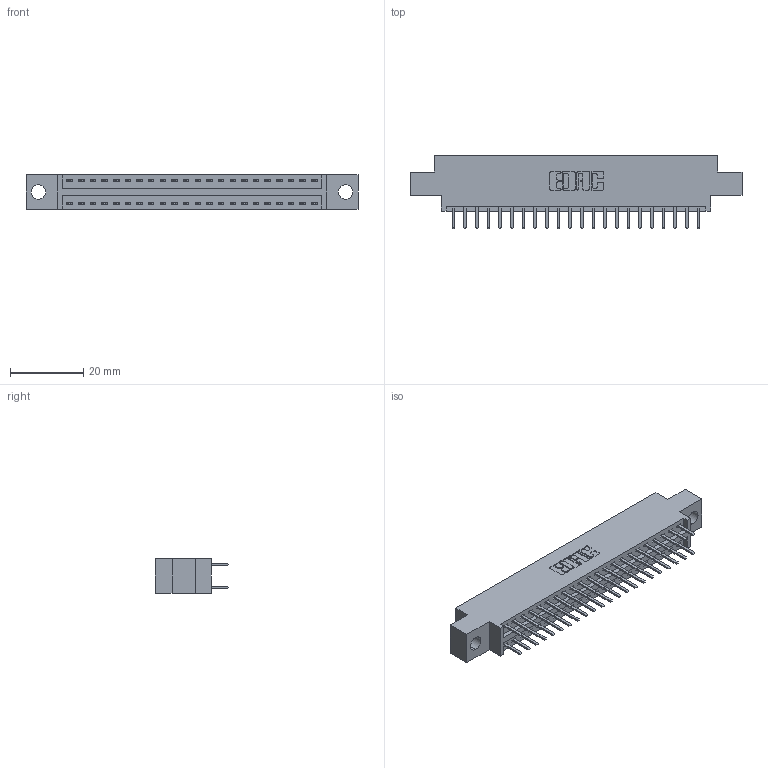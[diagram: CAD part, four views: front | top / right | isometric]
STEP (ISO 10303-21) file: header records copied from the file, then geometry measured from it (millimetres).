
FILE_DESCRIPTION (( 'STEP AP203' ), '1' );
FILE_NAME ('396-044-520-804.STEP', '2018-09-07T03:13:25', ( '' ), ( '' ), 'SwSTEP 2.0', 'SolidWorks 2016', '' );
FILE_SCHEMA (( 'CONFIG_CONTROL_DESIGN' ));
Length unit declared in the file: inch
Products named in the file (3): 346 Part_0.170 Offset - 0.156 Dia-TH; 345-292-001_345-293-120; 396-044-520-804
Assembly tree (45 placements, depth 2):
  396-044-520-804
    346 Part_0.170 Offset - 0.156 Dia-TH
    345-292-001_345-293-120  x44
Bounding box: 90.42 x 20.02 x 9.4 mm (x, y, z)
Volume: 8400.3 mm3; surface area: 11180.1 mm2
Topology: 45 solids, 45 shells, 2590 faces, 7513 edges, 4890 vertices
Faces by surface type: plane 1708, cylinder 882
Entity records: 17299 total; most frequent: CARTESIAN_POINT 2892, ORIENTED_EDGE 2814, DIRECTION 2587, EDGE_CURVE 1407, LINE 1183, VECTOR 1183, VERTEX_POINT 934, AXIS2_PLACEMENT_3D 702
